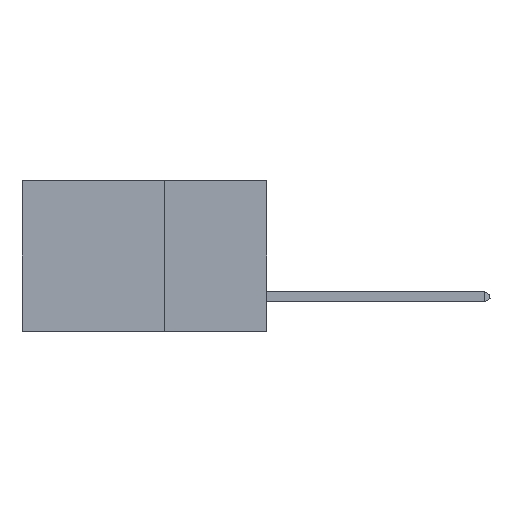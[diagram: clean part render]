
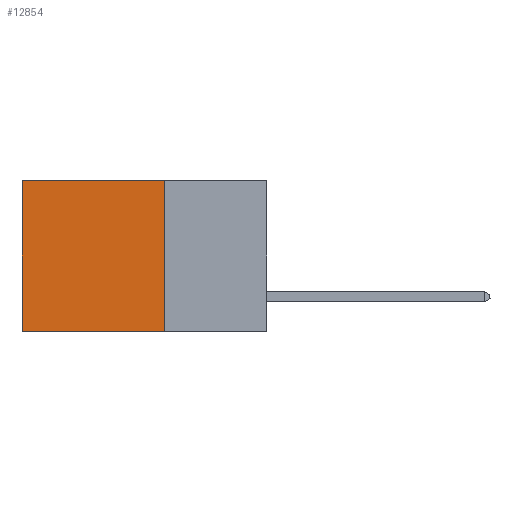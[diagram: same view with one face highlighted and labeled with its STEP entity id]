
A CAD part, left-side view. The second image highlights one B-rep face of the part: STEP entity #12854.
In plain terms, the highlighted planar face has unit normal (-1, 0, 0).
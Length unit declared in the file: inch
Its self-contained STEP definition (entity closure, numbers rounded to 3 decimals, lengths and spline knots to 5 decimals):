
#582 = VECTOR ( 'NONE', #24095, 39.37008 ) ;
#697 = VECTOR ( 'NONE', #12797, 39.37008 ) ;
#2775 = CARTESIAN_POINT ( 'NONE',  ( 0.2875, 0.6, 0. ) ) ;
#3130 = CARTESIAN_POINT ( 'NONE',  ( 0.2875, 0.6, 0. ) ) ;
#3457 = VERTEX_POINT ( 'NONE', #21121 ) ;
#4797 = ORIENTED_EDGE ( 'NONE', *, *, #16939, .T. ) ;
#4871 = DIRECTION ( 'NONE',  ( 0., 0., -1. ) ) ;
#5949 = CARTESIAN_POINT ( 'NONE',  ( 0.2875, 0.25, -0.37 ) ) ;
#6793 = EDGE_CURVE ( 'NONE', #12696, #3457, #8934, .T. ) ;
#7728 = FACE_OUTER_BOUND ( 'NONE', #23978, .T. ) ;
#8290 = ORIENTED_EDGE ( 'NONE', *, *, #11247, .T. ) ;
#8532 = CARTESIAN_POINT ( 'NONE',  ( 0.2875, 0.25, 0. ) ) ;
#8934 = LINE ( 'NONE', #9687, #582 ) ;
#8975 = PLANE ( 'NONE',  #11271 ) ;
#9687 = CARTESIAN_POINT ( 'NONE',  ( 0.2875, 0.25, 0. ) ) ;
#10288 = LINE ( 'NONE', #2775, #23524 ) ;
#11247 = EDGE_CURVE ( 'NONE', #12917, #26067, #10288, .T. ) ;
#11271 = AXIS2_PLACEMENT_3D ( 'NONE', #16986, #23387, #25204 ) ;
#12696 = VERTEX_POINT ( 'NONE', #8532 ) ;
#12797 = DIRECTION ( 'NONE',  ( 0., 1., 0. ) ) ;
#12854 = ADVANCED_FACE ( 'NONE', ( #7728 ), #8975, .F. ) ;
#12917 = VERTEX_POINT ( 'NONE', #3130 ) ;
#15506 = LINE ( 'NONE', #23227, #697 ) ;
#16565 = VECTOR ( 'NONE', #24760, 39.37008 ) ;
#16939 = EDGE_CURVE ( 'NONE', #12696, #12917, #15506, .T. ) ;
#16986 = CARTESIAN_POINT ( 'NONE',  ( 0.2875, 0.25, 0. ) ) ;
#21121 = CARTESIAN_POINT ( 'NONE',  ( 0.2875, 0.25, -0.37 ) ) ;
#21712 = CARTESIAN_POINT ( 'NONE',  ( 0.2875, 0.6, -0.37 ) ) ;
#21996 = EDGE_CURVE ( 'NONE', #3457, #26067, #23686, .T. ) ;
#22889 = ORIENTED_EDGE ( 'NONE', *, *, #21996, .F. ) ;
#23227 = CARTESIAN_POINT ( 'NONE',  ( 0.2875, 0.25, 0. ) ) ;
#23387 = DIRECTION ( 'NONE',  ( 1., 0., 0. ) ) ;
#23524 = VECTOR ( 'NONE', #4871, 39.37008 ) ;
#23686 = LINE ( 'NONE', #5949, #16565 ) ;
#23978 = EDGE_LOOP ( 'NONE', ( #8290, #22889, #26390, #4797 ) ) ;
#24095 = DIRECTION ( 'NONE',  ( 0., 0., -1. ) ) ;
#24760 = DIRECTION ( 'NONE',  ( 0., 1., 0. ) ) ;
#25204 = DIRECTION ( 'NONE',  ( 0., 0., -1. ) ) ;
#26067 = VERTEX_POINT ( 'NONE', #21712 ) ;
#26390 = ORIENTED_EDGE ( 'NONE', *, *, #6793, .F. ) ;
